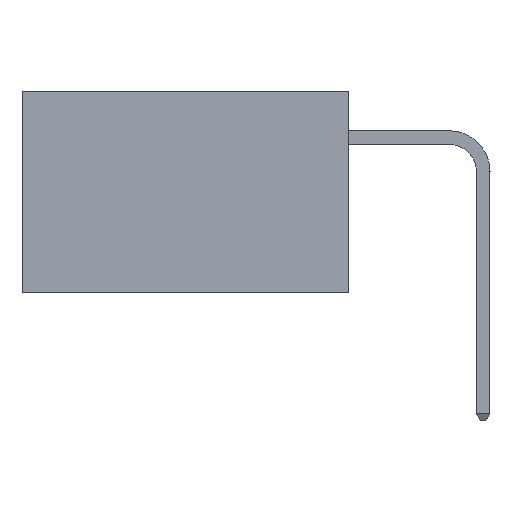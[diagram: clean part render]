
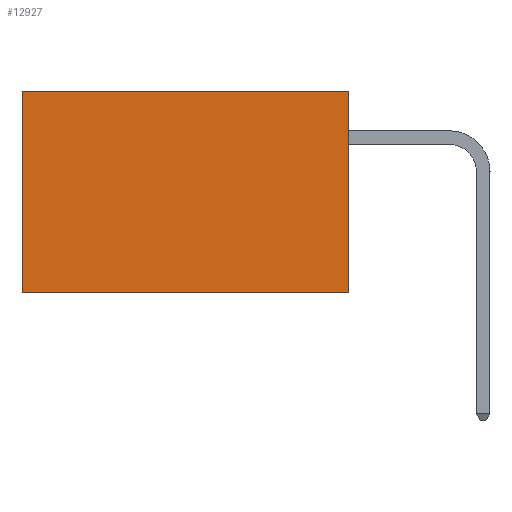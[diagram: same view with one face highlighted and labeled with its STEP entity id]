
A CAD part, left-side view. The second image highlights one B-rep face of the part: STEP entity #12927.
In plain terms, the highlighted planar face has unit normal (-1, 0, 0).
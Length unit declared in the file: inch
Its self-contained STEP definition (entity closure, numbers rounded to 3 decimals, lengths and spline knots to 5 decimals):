
#729 = EDGE_CURVE ( 'NONE', #9077, #14064, #5382, .T. ) ;
#1458 = PLANE ( 'NONE',  #7123 ) ;
#1939 = LINE ( 'NONE', #5705, #23533 ) ;
#3128 = LINE ( 'NONE', #10972, #8803 ) ;
#3630 = DIRECTION ( 'NONE',  ( 1., 0., 0. ) ) ;
#5382 = LINE ( 'NONE', #21025, #26782 ) ;
#5392 = CARTESIAN_POINT ( 'NONE',  ( 0.2875, 0.6, 0. ) ) ;
#5705 = CARTESIAN_POINT ( 'NONE',  ( 0.2875, 0., -0.37 ) ) ;
#6571 = VERTEX_POINT ( 'NONE', #25403 ) ;
#7123 = AXIS2_PLACEMENT_3D ( 'NONE', #7836, #3630, #18357 ) ;
#7836 = CARTESIAN_POINT ( 'NONE',  ( 0.2875, 0., 0. ) ) ;
#8545 = ORIENTED_EDGE ( 'NONE', *, *, #9470, .F. ) ;
#8803 = VECTOR ( 'NONE', #13025, 39.37008 ) ;
#8973 = FACE_OUTER_BOUND ( 'NONE', #25596, .T. ) ;
#9077 = VERTEX_POINT ( 'NONE', #25380 ) ;
#9470 = EDGE_CURVE ( 'NONE', #9077, #6571, #3128, .T. ) ;
#10972 = CARTESIAN_POINT ( 'NONE',  ( 0.2875, 0., 0. ) ) ;
#11166 = ORIENTED_EDGE ( 'NONE', *, *, #17345, .T. ) ;
#11453 = DIRECTION ( 'NONE',  ( 0., 1., 0. ) ) ;
#11573 = CARTESIAN_POINT ( 'NONE',  ( 0.2875, 0.6, -0.37 ) ) ;
#11978 = CARTESIAN_POINT ( 'NONE',  ( 0.2875, 0.6, 0. ) ) ;
#12922 = EDGE_CURVE ( 'NONE', #6571, #13445, #1939, .T. ) ;
#12927 = ADVANCED_FACE ( 'NONE', ( #8973 ), #1458, .F. ) ;
#13025 = DIRECTION ( 'NONE',  ( 0., 0., -1. ) ) ;
#13445 = VERTEX_POINT ( 'NONE', #11573 ) ;
#14064 = VERTEX_POINT ( 'NONE', #11978 ) ;
#14551 = ORIENTED_EDGE ( 'NONE', *, *, #729, .T. ) ;
#15547 = ORIENTED_EDGE ( 'NONE', *, *, #12922, .F. ) ;
#17345 = EDGE_CURVE ( 'NONE', #14064, #13445, #23509, .T. ) ;
#18357 = DIRECTION ( 'NONE',  ( 0., 0., -1. ) ) ;
#18745 = VECTOR ( 'NONE', #24003, 39.37008 ) ;
#21025 = CARTESIAN_POINT ( 'NONE',  ( 0.2875, 0., 0. ) ) ;
#22349 = DIRECTION ( 'NONE',  ( 0., 1., 0. ) ) ;
#23509 = LINE ( 'NONE', #5392, #18745 ) ;
#23533 = VECTOR ( 'NONE', #22349, 39.37008 ) ;
#24003 = DIRECTION ( 'NONE',  ( 0., 0., -1. ) ) ;
#25380 = CARTESIAN_POINT ( 'NONE',  ( 0.2875, 0., 0. ) ) ;
#25403 = CARTESIAN_POINT ( 'NONE',  ( 0.2875, 0., -0.37 ) ) ;
#25596 = EDGE_LOOP ( 'NONE', ( #11166, #15547, #8545, #14551 ) ) ;
#26782 = VECTOR ( 'NONE', #11453, 39.37008 ) ;
